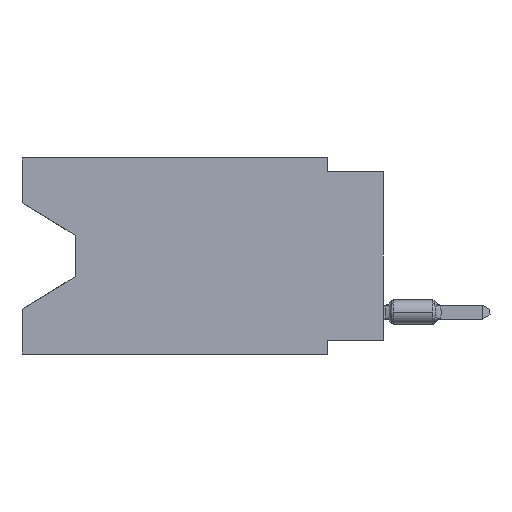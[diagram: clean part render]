
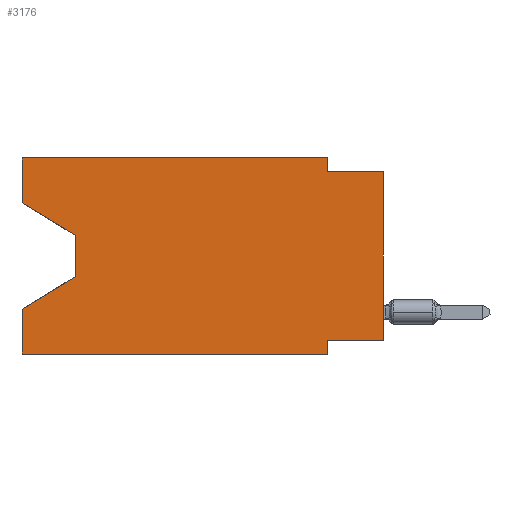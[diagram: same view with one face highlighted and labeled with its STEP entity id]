
A CAD part, left-side view. The second image highlights one B-rep face of the part: STEP entity #3176.
In plain terms, the highlighted planar face has unit normal (-1, 0, 0).
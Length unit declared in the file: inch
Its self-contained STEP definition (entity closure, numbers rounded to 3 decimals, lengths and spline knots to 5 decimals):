
#11 = ORIENTED_EDGE ( 'NONE', *, *, #11730, .F. ) ;
#81 = AXIS2_PLACEMENT_3D ( 'NONE', #11435, #2084, #5209 ) ;
#126 = LINE ( 'NONE', #4267, #8967 ) ;
#155 = ORIENTED_EDGE ( 'NONE', *, *, #11796, .T. ) ;
#294 = ORIENTED_EDGE ( 'NONE', *, *, #3677, .T. ) ;
#448 = EDGE_LOOP ( 'NONE', ( #8814, #6061, #10222, #6642, #155, #1965, #11, #294, #11750, #2678, #10221, #7488 ) ) ;
#587 = EDGE_CURVE ( 'NONE', #10319, #12713, #9223, .T. ) ;
#704 = VERTEX_POINT ( 'NONE', #9356 ) ;
#992 = DIRECTION ( 'NONE',  ( 0., 0., -1. ) ) ;
#998 = DIRECTION ( 'NONE',  ( 0., 0., -1. ) ) ;
#1083 = LINE ( 'NONE', #9343, #8433 ) ;
#1246 = LINE ( 'NONE', #11495, #8640 ) ;
#1544 = CARTESIAN_POINT ( 'NONE',  ( 0., 0.1, 0. ) ) ;
#1694 = VERTEX_POINT ( 'NONE', #7877 ) ;
#1859 = LINE ( 'NONE', #10042, #9058 ) ;
#1965 = ORIENTED_EDGE ( 'NONE', *, *, #6142, .F. ) ;
#2084 = DIRECTION ( 'NONE',  ( 1., 0., 0. ) ) ;
#2378 = CARTESIAN_POINT ( 'NONE',  ( 0., 0.1, -0.325 ) ) ;
#2510 = LINE ( 'NONE', #1544, #12222 ) ;
#2665 = DIRECTION ( 'NONE',  ( 0., -0.855, -0.519 ) ) ;
#2678 = ORIENTED_EDGE ( 'NONE', *, *, #5925, .F. ) ;
#2679 = VERTEX_POINT ( 'NONE', #9330 ) ;
#2690 = LINE ( 'NONE', #6858, #10239 ) ;
#3169 = DIRECTION ( 'NONE',  ( 0., 0., 1. ) ) ;
#3176 = ADVANCED_FACE ( 'NONE', ( #12455 ), #7263, .F. ) ;
#3623 = CARTESIAN_POINT ( 'NONE',  ( 0., 0.55, -0.212 ) ) ;
#3677 = EDGE_CURVE ( 'NONE', #704, #9375, #10600, .T. ) ;
#3869 = VECTOR ( 'NONE', #998, 39.37008 ) ;
#3931 = EDGE_CURVE ( 'NONE', #4558, #7903, #1859, .T. ) ;
#4267 = CARTESIAN_POINT ( 'NONE',  ( 0., 0.645, 0. ) ) ;
#4500 = EDGE_CURVE ( 'NONE', #9911, #12713, #126, .T. ) ;
#4558 = VERTEX_POINT ( 'NONE', #8787 ) ;
#4902 = EDGE_CURVE ( 'NONE', #4558, #5624, #10414, .T. ) ;
#4974 = DIRECTION ( 'NONE',  ( 0., 1., 0. ) ) ;
#5202 = CARTESIAN_POINT ( 'NONE',  ( 0., 0., 0. ) ) ;
#5209 = DIRECTION ( 'NONE',  ( 0., 0., -1. ) ) ;
#5220 = CARTESIAN_POINT ( 'NONE',  ( 0., 0.645, 0. ) ) ;
#5624 = VERTEX_POINT ( 'NONE', #12080 ) ;
#5925 = EDGE_CURVE ( 'NONE', #10887, #2679, #2510, .T. ) ;
#6061 = ORIENTED_EDGE ( 'NONE', *, *, #13470, .T. ) ;
#6113 = CARTESIAN_POINT ( 'NONE',  ( 0., 0.1, -0.35 ) ) ;
#6142 = EDGE_CURVE ( 'NONE', #13190, #1694, #7274, .T. ) ;
#6268 = DIRECTION ( 'NONE',  ( 0., -1., 0. ) ) ;
#6434 = DIRECTION ( 'NONE',  ( 0., 0., 1. ) ) ;
#6450 = EDGE_CURVE ( 'NONE', #5624, #10887, #2690, .T. ) ;
#6642 = ORIENTED_EDGE ( 'NONE', *, *, #4500, .F. ) ;
#6674 = DIRECTION ( 'NONE',  ( 0., 0., -1. ) ) ;
#6855 = CARTESIAN_POINT ( 'NONE',  ( 0., 0.645, -0.35 ) ) ;
#6858 = CARTESIAN_POINT ( 'NONE',  ( 0., 0.645, 0. ) ) ;
#7261 = CARTESIAN_POINT ( 'NONE',  ( 0., 0.645, -0.26975 ) ) ;
#7263 = PLANE ( 'NONE',  #81 ) ;
#7274 = LINE ( 'NONE', #6113, #11756 ) ;
#7488 = ORIENTED_EDGE ( 'NONE', *, *, #4902, .F. ) ;
#7877 = CARTESIAN_POINT ( 'NONE',  ( 0., 0.1, -0.35 ) ) ;
#7903 = VERTEX_POINT ( 'NONE', #12074 ) ;
#8056 = LINE ( 'NONE', #13174, #13008 ) ;
#8379 = LINE ( 'NONE', #10356, #3869 ) ;
#8433 = VECTOR ( 'NONE', #6268, 39.37008 ) ;
#8467 = CARTESIAN_POINT ( 'NONE',  ( 0., 0., -0.025 ) ) ;
#8621 = VECTOR ( 'NONE', #6434, 39.37008 ) ;
#8640 = VECTOR ( 'NONE', #12710, 39.37008 ) ;
#8787 = CARTESIAN_POINT ( 'NONE',  ( 0., 0.645, -0.08025 ) ) ;
#8814 = ORIENTED_EDGE ( 'NONE', *, *, #3931, .T. ) ;
#8967 = VECTOR ( 'NONE', #13492, 39.37008 ) ;
#9058 = VECTOR ( 'NONE', #2665, 39.37008 ) ;
#9143 = CARTESIAN_POINT ( 'NONE',  ( 0., 0.1, 0. ) ) ;
#9223 = LINE ( 'NONE', #10313, #11164 ) ;
#9330 = CARTESIAN_POINT ( 'NONE',  ( 0., 0.1, -0.025 ) ) ;
#9343 = CARTESIAN_POINT ( 'NONE',  ( 0., 0.645, -0.35 ) ) ;
#9356 = CARTESIAN_POINT ( 'NONE',  ( 0., 0., -0.325 ) ) ;
#9375 = VERTEX_POINT ( 'NONE', #8467 ) ;
#9838 = VECTOR ( 'NONE', #3169, 39.37008 ) ;
#9911 = VERTEX_POINT ( 'NONE', #6855 ) ;
#10042 = CARTESIAN_POINT ( 'NONE',  ( 0., 0.645, -0.08025 ) ) ;
#10221 = ORIENTED_EDGE ( 'NONE', *, *, #6450, .F. ) ;
#10222 = ORIENTED_EDGE ( 'NONE', *, *, #587, .T. ) ;
#10239 = VECTOR ( 'NONE', #11161, 39.37008 ) ;
#10285 = EDGE_CURVE ( 'NONE', #2679, #9375, #1246, .T. ) ;
#10313 = CARTESIAN_POINT ( 'NONE',  ( 0., 0.55, -0.212 ) ) ;
#10319 = VERTEX_POINT ( 'NONE', #3623 ) ;
#10356 = CARTESIAN_POINT ( 'NONE',  ( 0., 0.55, -0.138 ) ) ;
#10414 = LINE ( 'NONE', #5220, #9838 ) ;
#10600 = LINE ( 'NONE', #5202, #8621 ) ;
#10887 = VERTEX_POINT ( 'NONE', #9143 ) ;
#11161 = DIRECTION ( 'NONE',  ( 0., -1., 0. ) ) ;
#11164 = VECTOR ( 'NONE', #13186, 39.37008 ) ;
#11435 = CARTESIAN_POINT ( 'NONE',  ( 0., 0.645, 0. ) ) ;
#11495 = CARTESIAN_POINT ( 'NONE',  ( 0., 0., -0.025 ) ) ;
#11730 = EDGE_CURVE ( 'NONE', #704, #13190, #8056, .T. ) ;
#11750 = ORIENTED_EDGE ( 'NONE', *, *, #10285, .F. ) ;
#11756 = VECTOR ( 'NONE', #992, 39.37008 ) ;
#11796 = EDGE_CURVE ( 'NONE', #9911, #1694, #1083, .T. ) ;
#12074 = CARTESIAN_POINT ( 'NONE',  ( 0., 0.55, -0.138 ) ) ;
#12080 = CARTESIAN_POINT ( 'NONE',  ( 0., 0.645, 0. ) ) ;
#12222 = VECTOR ( 'NONE', #6674, 39.37008 ) ;
#12455 = FACE_OUTER_BOUND ( 'NONE', #448, .T. ) ;
#12710 = DIRECTION ( 'NONE',  ( 0., -1., 0. ) ) ;
#12713 = VERTEX_POINT ( 'NONE', #7261 ) ;
#13008 = VECTOR ( 'NONE', #4974, 39.37008 ) ;
#13174 = CARTESIAN_POINT ( 'NONE',  ( 0., 0., -0.325 ) ) ;
#13186 = DIRECTION ( 'NONE',  ( 0., 0.855, -0.519 ) ) ;
#13190 = VERTEX_POINT ( 'NONE', #2378 ) ;
#13470 = EDGE_CURVE ( 'NONE', #7903, #10319, #8379, .T. ) ;
#13492 = DIRECTION ( 'NONE',  ( 0., 0., 1. ) ) ;
